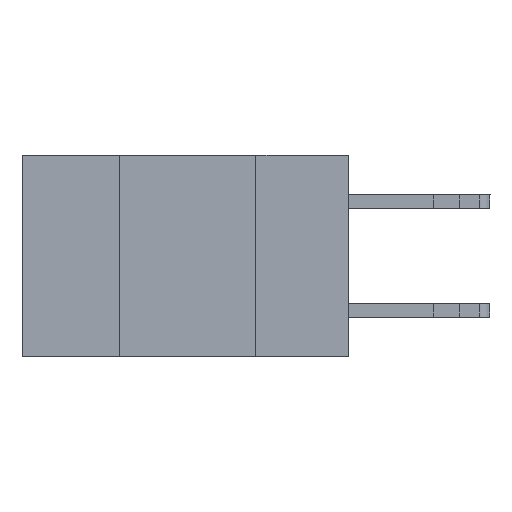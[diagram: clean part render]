
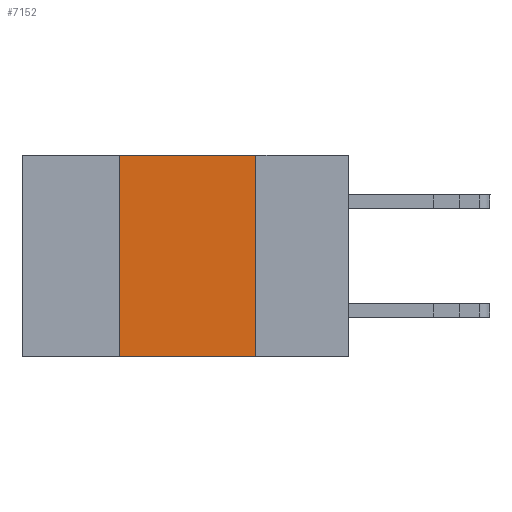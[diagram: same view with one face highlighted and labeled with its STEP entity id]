
A CAD part, left-side view. The second image highlights one B-rep face of the part: STEP entity #7152.
In plain terms, the highlighted planar face has unit normal (-1, 0, 0).
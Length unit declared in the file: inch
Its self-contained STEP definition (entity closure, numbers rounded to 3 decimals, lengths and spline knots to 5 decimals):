
#251 = CARTESIAN_POINT ( 'NONE',  ( 0., 0.42, 0. ) ) ;
#537 = ORIENTED_EDGE ( 'NONE', *, *, #10876, .T. ) ;
#774 = LINE ( 'NONE', #5660, #1657 ) ;
#1041 = CARTESIAN_POINT ( 'NONE',  ( 0., 0.17, -0.37 ) ) ;
#1438 = CARTESIAN_POINT ( 'NONE',  ( 0., 0.42, -0.37 ) ) ;
#1657 = VECTOR ( 'NONE', #4445, 39.37008 ) ;
#2259 = EDGE_CURVE ( 'NONE', #14489, #13973, #12649, .T. ) ;
#2626 = ORIENTED_EDGE ( 'NONE', *, *, #2259, .F. ) ;
#2827 = DIRECTION ( 'NONE',  ( 0., -1., 0. ) ) ;
#3140 = EDGE_CURVE ( 'NONE', #13973, #7192, #774, .T. ) ;
#3714 = VERTEX_POINT ( 'NONE', #1438 ) ;
#4313 = PLANE ( 'NONE',  #14563 ) ;
#4426 = CARTESIAN_POINT ( 'NONE',  ( 0., 0.17, 0. ) ) ;
#4445 = DIRECTION ( 'NONE',  ( 0., 0., -1. ) ) ;
#5054 = ORIENTED_EDGE ( 'NONE', *, *, #10067, .F. ) ;
#5441 = DIRECTION ( 'NONE',  ( 1., 0., 0. ) ) ;
#5660 = CARTESIAN_POINT ( 'NONE',  ( 0., 0.17, 0. ) ) ;
#6508 = DIRECTION ( 'NONE',  ( 0., 0., 1. ) ) ;
#6665 = LINE ( 'NONE', #251, #11094 ) ;
#6728 = CARTESIAN_POINT ( 'NONE',  ( 0., 0.6, 0. ) ) ;
#7152 = ADVANCED_FACE ( 'NONE', ( #8084 ), #4313, .F. ) ;
#7192 = VERTEX_POINT ( 'NONE', #1041 ) ;
#7717 = LINE ( 'NONE', #11486, #9585 ) ;
#8084 = FACE_OUTER_BOUND ( 'NONE', #8747, .T. ) ;
#8747 = EDGE_LOOP ( 'NONE', ( #9324, #2626, #5054, #537 ) ) ;
#9324 = ORIENTED_EDGE ( 'NONE', *, *, #3140, .F. ) ;
#9585 = VECTOR ( 'NONE', #2827, 39.37008 ) ;
#10067 = EDGE_CURVE ( 'NONE', #3714, #14489, #6665, .T. ) ;
#10876 = EDGE_CURVE ( 'NONE', #3714, #7192, #7717, .T. ) ;
#11094 = VECTOR ( 'NONE', #6508, 39.37008 ) ;
#11365 = DIRECTION ( 'NONE',  ( 0., -1., 0. ) ) ;
#11486 = CARTESIAN_POINT ( 'NONE',  ( 0., 0.6, -0.37 ) ) ;
#12645 = VECTOR ( 'NONE', #11365, 39.37008 ) ;
#12649 = LINE ( 'NONE', #13848, #12645 ) ;
#12813 = DIRECTION ( 'NONE',  ( 0., 0., -1. ) ) ;
#13848 = CARTESIAN_POINT ( 'NONE',  ( 0., 0.6, 0. ) ) ;
#13973 = VERTEX_POINT ( 'NONE', #4426 ) ;
#14489 = VERTEX_POINT ( 'NONE', #15809 ) ;
#14563 = AXIS2_PLACEMENT_3D ( 'NONE', #6728, #5441, #12813 ) ;
#15809 = CARTESIAN_POINT ( 'NONE',  ( 0., 0.42, 0. ) ) ;
